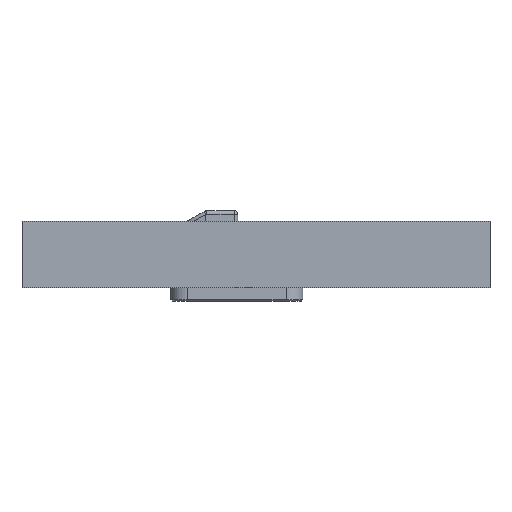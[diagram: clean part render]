
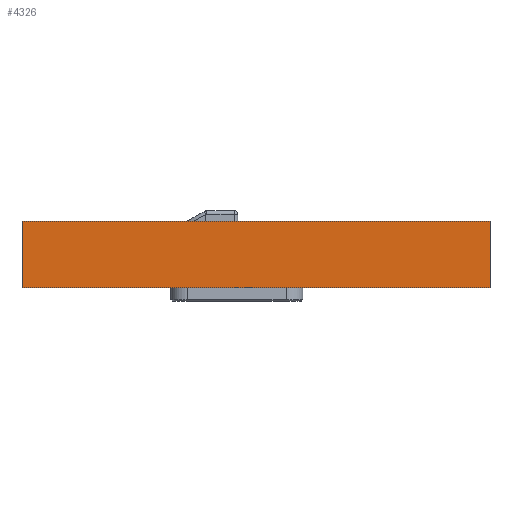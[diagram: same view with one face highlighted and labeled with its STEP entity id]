
A CAD part, left-side view. The second image highlights one B-rep face of the part: STEP entity #4326.
In plain terms, the highlighted planar face has unit normal (-1, 0, 0).
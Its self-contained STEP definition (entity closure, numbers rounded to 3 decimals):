
#4326 = ADVANCED_FACE('',(#4327),#4361,.F.);
#4327 = FACE_BOUND('',#4328,.F.);
#4328 = EDGE_LOOP('',(#4329,#4339,#4347,#4355));
#4329 = ORIENTED_EDGE('',*,*,#4330,.F.);
#4330 = EDGE_CURVE('',#4331,#4333,#4335,.T.);
#4331 = VERTEX_POINT('',#4332);
#4332 = CARTESIAN_POINT('',(0.,0.,0.));
#4333 = VERTEX_POINT('',#4334);
#4334 = CARTESIAN_POINT('',(0.,0.,10.));
#4335 = LINE('',#4336,#4337);
#4336 = CARTESIAN_POINT('',(0.,0.,0.));
#4337 = VECTOR('',#4338,1.);
#4338 = DIRECTION('',(0.,0.,1.));
#4339 = ORIENTED_EDGE('',*,*,#4340,.T.);
#4340 = EDGE_CURVE('',#4331,#4341,#4343,.T.);
#4341 = VERTEX_POINT('',#4342);
#4342 = CARTESIAN_POINT('',(0.,70.,0.));
#4343 = LINE('',#4344,#4345);
#4344 = CARTESIAN_POINT('',(0.,0.,0.));
#4345 = VECTOR('',#4346,1.);
#4346 = DIRECTION('',(-0.,1.,0.));
#4347 = ORIENTED_EDGE('',*,*,#4348,.T.);
#4348 = EDGE_CURVE('',#4341,#4349,#4351,.T.);
#4349 = VERTEX_POINT('',#4350);
#4350 = CARTESIAN_POINT('',(0.,70.,10.));
#4351 = LINE('',#4352,#4353);
#4352 = CARTESIAN_POINT('',(0.,70.,0.));
#4353 = VECTOR('',#4354,1.);
#4354 = DIRECTION('',(0.,0.,1.));
#4355 = ORIENTED_EDGE('',*,*,#4356,.F.);
#4356 = EDGE_CURVE('',#4333,#4349,#4357,.T.);
#4357 = LINE('',#4358,#4359);
#4358 = CARTESIAN_POINT('',(0.,0.,10.));
#4359 = VECTOR('',#4360,1.);
#4360 = DIRECTION('',(-0.,1.,0.));
#4361 = PLANE('',#4362);
#4362 = AXIS2_PLACEMENT_3D('',#4363,#4364,#4365);
#4363 = CARTESIAN_POINT('',(0.,0.,0.));
#4364 = DIRECTION('',(1.,0.,-0.));
#4365 = DIRECTION('',(0.,0.,1.));
